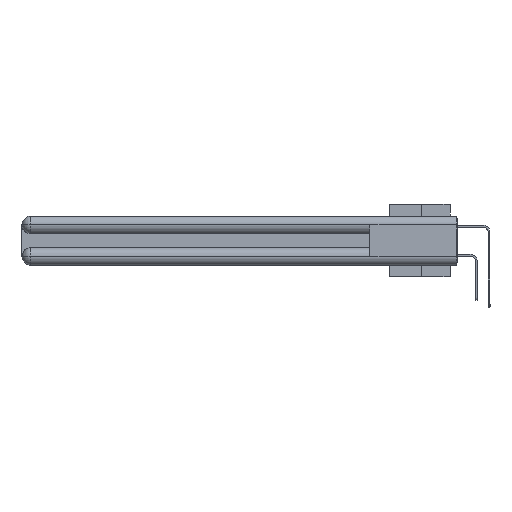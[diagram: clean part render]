
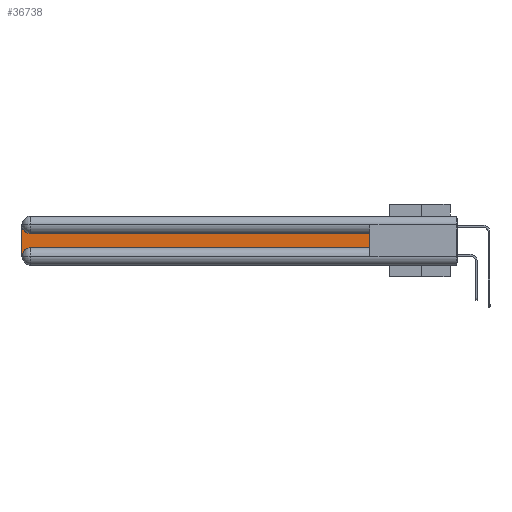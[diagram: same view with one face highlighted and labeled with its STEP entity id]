
A CAD part, left-side view. The second image highlights one B-rep face of the part: STEP entity #36738.
In plain terms, the highlighted planar face has unit normal (-1, 0, 0).
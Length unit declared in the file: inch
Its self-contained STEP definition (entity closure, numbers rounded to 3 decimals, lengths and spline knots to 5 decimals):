
#1260 = VERTEX_POINT ( 'NONE', #22389 ) ;
#2165 = LINE ( 'NONE', #29492, #33105 ) ;
#3857 = ORIENTED_EDGE ( 'NONE', *, *, #16947, .T. ) ;
#4427 = CARTESIAN_POINT ( 'NONE',  ( 0.075, 0.6, -0.2175 ) ) ;
#4701 = AXIS2_PLACEMENT_3D ( 'NONE', #27982, #37825, #32186 ) ;
#5019 = DIRECTION ( 'NONE',  ( 0., 0., 1. ) ) ;
#5377 = CIRCLE ( 'NONE', #4701, 0.06 ) ;
#6377 = EDGE_CURVE ( 'NONE', #27519, #31228, #5377, .T. ) ;
#6619 = DIRECTION ( 'NONE',  ( 0., 0., -1. ) ) ;
#7853 = CARTESIAN_POINT ( 'NONE',  ( 0.075, 3., -0.1225 ) ) ;
#8226 = VERTEX_POINT ( 'NONE', #4427 ) ;
#11497 = DIRECTION ( 'NONE',  ( 0., -1., 0. ) ) ;
#11595 = VECTOR ( 'NONE', #27043, 39.37008 ) ;
#11839 = LINE ( 'NONE', #39679, #25759 ) ;
#12297 = CARTESIAN_POINT ( 'NONE',  ( 0.075, 2.94, -0.2775 ) ) ;
#13800 = CARTESIAN_POINT ( 'NONE',  ( 0.075, 3., -0.0625 ) ) ;
#14243 = ORIENTED_EDGE ( 'NONE', *, *, #29336, .T. ) ;
#14739 = VECTOR ( 'NONE', #5019, 39.37008 ) ;
#14855 = ORIENTED_EDGE ( 'NONE', *, *, #29488, .T. ) ;
#16072 = EDGE_LOOP ( 'NONE', ( #31344, #25553, #24156, #14855, #14243, #3857 ) ) ;
#16126 = CARTESIAN_POINT ( 'NONE',  ( 0.075, 0.6, -0.1225 ) ) ;
#16947 = EDGE_CURVE ( 'NONE', #8226, #30721, #26270, .T. ) ;
#17436 = EDGE_CURVE ( 'NONE', #30721, #27519, #11839, .T. ) ;
#18172 = DIRECTION ( 'NONE',  ( 1., 0., 0. ) ) ;
#18186 = EDGE_CURVE ( 'NONE', #31228, #33496, #33297, .T. ) ;
#20192 = CARTESIAN_POINT ( 'NONE',  ( 0.075, 3., -0.2175 ) ) ;
#20198 = DIRECTION ( 'NONE',  ( 0., 0., -1. ) ) ;
#22389 = CARTESIAN_POINT ( 'NONE',  ( 0.075, 2.94, -0.2175 ) ) ;
#24156 = ORIENTED_EDGE ( 'NONE', *, *, #18186, .T. ) ;
#25553 = ORIENTED_EDGE ( 'NONE', *, *, #6377, .T. ) ;
#25759 = VECTOR ( 'NONE', #27184, 39.37008 ) ;
#26024 = CIRCLE ( 'NONE', #39552, 0.06 ) ;
#26058 = PLANE ( 'NONE',  #37875 ) ;
#26270 = LINE ( 'NONE', #38565, #14739 ) ;
#27043 = DIRECTION ( 'NONE',  ( 0., 0., -1. ) ) ;
#27184 = DIRECTION ( 'NONE',  ( 0., 1., 0. ) ) ;
#27519 = VERTEX_POINT ( 'NONE', #38385 ) ;
#27982 = CARTESIAN_POINT ( 'NONE',  ( 0.075, 2.94, -0.0625 ) ) ;
#29336 = EDGE_CURVE ( 'NONE', #1260, #8226, #2165, .T. ) ;
#29488 = EDGE_CURVE ( 'NONE', #33496, #1260, #26024, .T. ) ;
#29492 = CARTESIAN_POINT ( 'NONE',  ( 0.075, 0.6, -0.2175 ) ) ;
#29693 = DIRECTION ( 'NONE',  ( 1., 0., 0. ) ) ;
#30721 = VERTEX_POINT ( 'NONE', #16126 ) ;
#31228 = VERTEX_POINT ( 'NONE', #13800 ) ;
#31264 = CARTESIAN_POINT ( 'NONE',  ( 0.075, 3., -0.2775 ) ) ;
#31344 = ORIENTED_EDGE ( 'NONE', *, *, #17436, .T. ) ;
#32186 = DIRECTION ( 'NONE',  ( 0., 0., -1. ) ) ;
#33105 = VECTOR ( 'NONE', #11497, 39.37008 ) ;
#33297 = LINE ( 'NONE', #20192, #11595 ) ;
#33496 = VERTEX_POINT ( 'NONE', #31264 ) ;
#35510 = FACE_OUTER_BOUND ( 'NONE', #16072, .T. ) ;
#36738 = ADVANCED_FACE ( 'NONE', ( #35510 ), #26058, .F. ) ;
#37825 = DIRECTION ( 'NONE',  ( 1., 0., 0. ) ) ;
#37875 = AXIS2_PLACEMENT_3D ( 'NONE', #7853, #29693, #20198 ) ;
#38385 = CARTESIAN_POINT ( 'NONE',  ( 0.075, 2.94, -0.1225 ) ) ;
#38565 = CARTESIAN_POINT ( 'NONE',  ( 0.075, 0.6, -0.2175 ) ) ;
#39552 = AXIS2_PLACEMENT_3D ( 'NONE', #12297, #18172, #6619 ) ;
#39679 = CARTESIAN_POINT ( 'NONE',  ( 0.075, 0.6, -0.1225 ) ) ;
